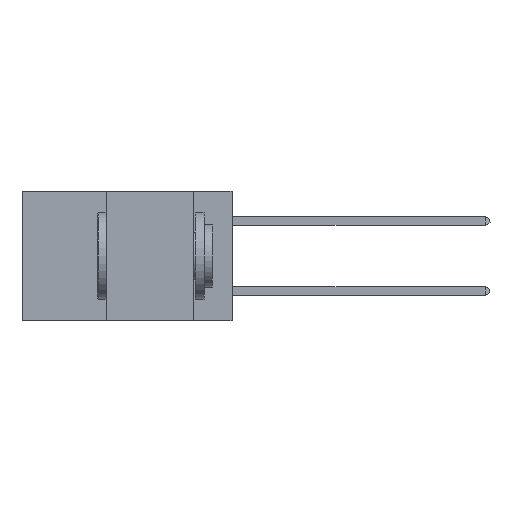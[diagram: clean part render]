
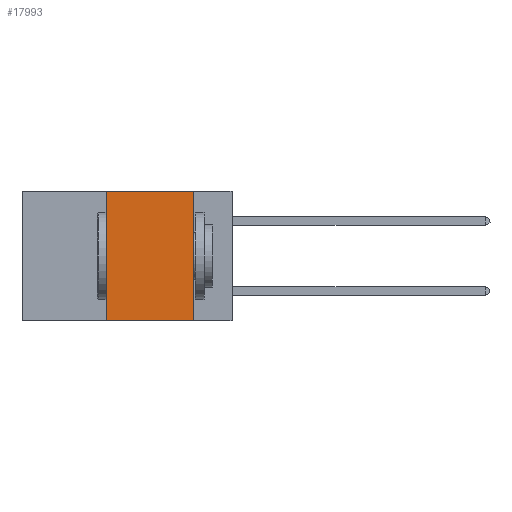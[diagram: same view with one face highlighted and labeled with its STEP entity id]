
A CAD part, left-side view. The second image highlights one B-rep face of the part: STEP entity #17993.
In plain terms, the highlighted planar face has unit normal (-1, 0, 0).
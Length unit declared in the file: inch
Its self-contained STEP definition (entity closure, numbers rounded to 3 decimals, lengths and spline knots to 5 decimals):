
#288 = PLANE ( 'NONE',  #11653 ) ;
#834 = CARTESIAN_POINT ( 'NONE',  ( 0., 0.36, -0.37 ) ) ;
#1179 = EDGE_LOOP ( 'NONE', ( #1290, #7376, #9423, #4698 ) ) ;
#1290 = ORIENTED_EDGE ( 'NONE', *, *, #16026, .F. ) ;
#1919 = LINE ( 'NONE', #12788, #14738 ) ;
#3990 = LINE ( 'NONE', #13864, #5612 ) ;
#4318 = VECTOR ( 'NONE', #16781, 39.37008 ) ;
#4698 = ORIENTED_EDGE ( 'NONE', *, *, #7788, .T. ) ;
#5066 = DIRECTION ( 'NONE',  ( 0., -1., 0. ) ) ;
#5326 = DIRECTION ( 'NONE',  ( 0., 0., 1. ) ) ;
#5612 = VECTOR ( 'NONE', #5066, 39.37008 ) ;
#6136 = VERTEX_POINT ( 'NONE', #15664 ) ;
#7376 = ORIENTED_EDGE ( 'NONE', *, *, #18466, .F. ) ;
#7398 = DIRECTION ( 'NONE',  ( 0., 0., -1. ) ) ;
#7788 = EDGE_CURVE ( 'NONE', #12250, #6136, #10784, .T. ) ;
#8418 = EDGE_CURVE ( 'NONE', #12250, #18768, #1919, .T. ) ;
#8777 = CARTESIAN_POINT ( 'NONE',  ( 0., 0.11, 0. ) ) ;
#9423 = ORIENTED_EDGE ( 'NONE', *, *, #8418, .F. ) ;
#10720 = FACE_OUTER_BOUND ( 'NONE', #1179, .T. ) ;
#10784 = LINE ( 'NONE', #12759, #4318 ) ;
#10986 = DIRECTION ( 'NONE',  ( 0., 0., -1. ) ) ;
#11653 = AXIS2_PLACEMENT_3D ( 'NONE', #16785, #18295, #10986 ) ;
#12250 = VERTEX_POINT ( 'NONE', #834 ) ;
#12759 = CARTESIAN_POINT ( 'NONE',  ( 0., 0.6, -0.37 ) ) ;
#12788 = CARTESIAN_POINT ( 'NONE',  ( 0., 0.36, 0. ) ) ;
#13111 = CARTESIAN_POINT ( 'NONE',  ( 0., 0.36, 0. ) ) ;
#13136 = LINE ( 'NONE', #8777, #15612 ) ;
#13864 = CARTESIAN_POINT ( 'NONE',  ( 0., 0.6, 0. ) ) ;
#14738 = VECTOR ( 'NONE', #5326, 39.37008 ) ;
#15595 = CARTESIAN_POINT ( 'NONE',  ( 0., 0.11, 0. ) ) ;
#15612 = VECTOR ( 'NONE', #7398, 39.37008 ) ;
#15664 = CARTESIAN_POINT ( 'NONE',  ( 0., 0.11, -0.37 ) ) ;
#16026 = EDGE_CURVE ( 'NONE', #18623, #6136, #13136, .T. ) ;
#16781 = DIRECTION ( 'NONE',  ( 0., -1., 0. ) ) ;
#16785 = CARTESIAN_POINT ( 'NONE',  ( 0., 0.6, 0. ) ) ;
#17993 = ADVANCED_FACE ( 'NONE', ( #10720 ), #288, .F. ) ;
#18295 = DIRECTION ( 'NONE',  ( 1., 0., 0. ) ) ;
#18466 = EDGE_CURVE ( 'NONE', #18768, #18623, #3990, .T. ) ;
#18623 = VERTEX_POINT ( 'NONE', #15595 ) ;
#18768 = VERTEX_POINT ( 'NONE', #13111 ) ;
